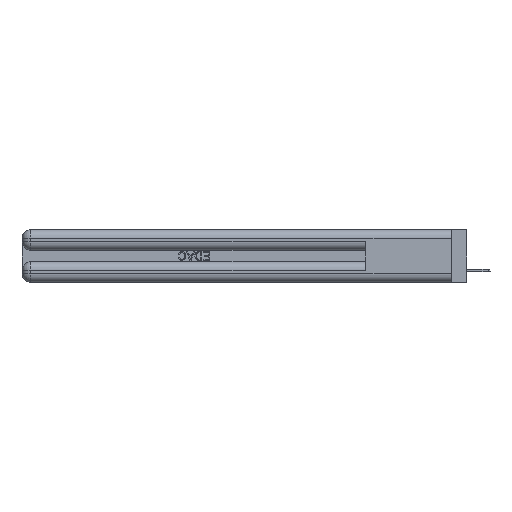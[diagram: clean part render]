
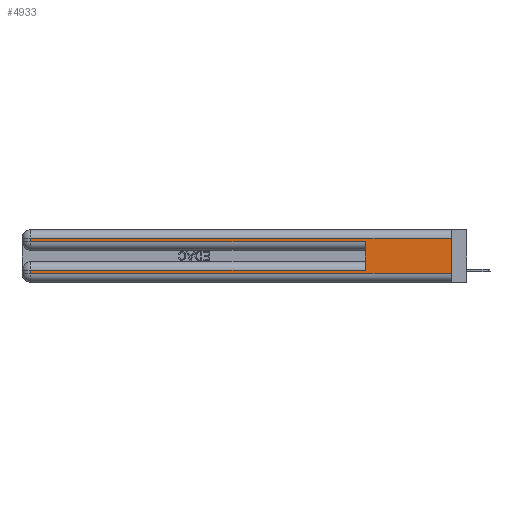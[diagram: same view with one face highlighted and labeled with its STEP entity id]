
A CAD part, left-side view. The second image highlights one B-rep face of the part: STEP entity #4933.
In plain terms, the highlighted planar face has unit normal (-1, 0, 0).
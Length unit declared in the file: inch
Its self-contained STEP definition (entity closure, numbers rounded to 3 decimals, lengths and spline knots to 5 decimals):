
#1 = FACE_OUTER_BOUND ( 'NONE', #5057, .T. ) ;
#409 = VERTEX_POINT ( 'NONE', #12928 ) ;
#585 = VERTEX_POINT ( 'NONE', #13416 ) ;
#693 = EDGE_CURVE ( 'NONE', #15766, #15949, #33570, .T. ) ;
#899 = VECTOR ( 'NONE', #7344, 39.37008 ) ;
#920 = ORIENTED_EDGE ( 'NONE', *, *, #13534, .T. ) ;
#3153 = ORIENTED_EDGE ( 'NONE', *, *, #22702, .F. ) ;
#3956 = DIRECTION ( 'NONE',  ( 0., 0., 1. ) ) ;
#4933 = ADVANCED_FACE ( 'NONE', ( #1 ), #30703, .F. ) ;
#5057 = EDGE_LOOP ( 'NONE', ( #3153, #31452, #42704, #10054, #16889, #920, #41786, #15667 ) ) ;
#5672 = CARTESIAN_POINT ( 'NONE',  ( 0., 0., 0.085 ) ) ;
#6010 = VECTOR ( 'NONE', #7551, 39.37008 ) ;
#7015 = EDGE_CURVE ( 'NONE', #585, #23819, #20651, .T. ) ;
#7344 = DIRECTION ( 'NONE',  ( 0., 1., 0. ) ) ;
#7551 = DIRECTION ( 'NONE',  ( 0., 0., -1. ) ) ;
#9021 = LINE ( 'NONE', #29545, #44874 ) ;
#9796 = LINE ( 'NONE', #39107, #19837 ) ;
#10054 = ORIENTED_EDGE ( 'NONE', *, *, #35506, .T. ) ;
#10888 = EDGE_CURVE ( 'NONE', #15949, #28149, #39753, .T. ) ;
#11546 = CARTESIAN_POINT ( 'NONE',  ( 0., 0., 0.06 ) ) ;
#11965 = DIRECTION ( 'NONE',  ( 0., -1., 0. ) ) ;
#12458 = CARTESIAN_POINT ( 'NONE',  ( 0., 0., 0.31 ) ) ;
#12928 = CARTESIAN_POINT ( 'NONE',  ( 0., 2.94, 0.085 ) ) ;
#13416 = CARTESIAN_POINT ( 'NONE',  ( 0., 0.6, 0.085 ) ) ;
#13534 = EDGE_CURVE ( 'NONE', #585, #409, #28419, .T. ) ;
#14005 = CARTESIAN_POINT ( 'NONE',  ( 0., 0., 0.31 ) ) ;
#14333 = CARTESIAN_POINT ( 'NONE',  ( 0., 0.6, 0.145 ) ) ;
#15351 = AXIS2_PLACEMENT_3D ( 'NONE', #30994, #27719, #19470 ) ;
#15667 = ORIENTED_EDGE ( 'NONE', *, *, #41146, .T. ) ;
#15766 = VERTEX_POINT ( 'NONE', #12458 ) ;
#15949 = VERTEX_POINT ( 'NONE', #16830 ) ;
#16182 = VECTOR ( 'NONE', #16986, 39.37008 ) ;
#16830 = CARTESIAN_POINT ( 'NONE',  ( 0., 2.94, 0.31 ) ) ;
#16889 = ORIENTED_EDGE ( 'NONE', *, *, #7015, .F. ) ;
#16986 = DIRECTION ( 'NONE',  ( 0., -1., 0. ) ) ;
#17973 = VECTOR ( 'NONE', #23342, 39.37008 ) ;
#18191 = LINE ( 'NONE', #39471, #6010 ) ;
#19470 = DIRECTION ( 'NONE',  ( 0., 0., -1. ) ) ;
#19837 = VECTOR ( 'NONE', #31599, 39.37008 ) ;
#20651 = LINE ( 'NONE', #14333, #37131 ) ;
#21470 = VERTEX_POINT ( 'NONE', #31205 ) ;
#21498 = CARTESIAN_POINT ( 'NONE',  ( 0., 2.94, 0.37 ) ) ;
#22702 = EDGE_CURVE ( 'NONE', #15766, #26576, #9796, .T. ) ;
#23342 = DIRECTION ( 'NONE',  ( 0., 1., 0. ) ) ;
#23608 = CARTESIAN_POINT ( 'NONE',  ( 0., 0., 0.06 ) ) ;
#23819 = VERTEX_POINT ( 'NONE', #34543 ) ;
#26576 = VERTEX_POINT ( 'NONE', #11546 ) ;
#27719 = DIRECTION ( 'NONE',  ( 1., 0., 0. ) ) ;
#28149 = VERTEX_POINT ( 'NONE', #31568 ) ;
#28419 = LINE ( 'NONE', #5672, #17973 ) ;
#29545 = CARTESIAN_POINT ( 'NONE',  ( 0., 0., 0.285 ) ) ;
#30703 = PLANE ( 'NONE',  #15351 ) ;
#30994 = CARTESIAN_POINT ( 'NONE',  ( 0., 0., 0.37 ) ) ;
#31205 = CARTESIAN_POINT ( 'NONE',  ( 0., 2.94, 0.06 ) ) ;
#31452 = ORIENTED_EDGE ( 'NONE', *, *, #693, .T. ) ;
#31568 = CARTESIAN_POINT ( 'NONE',  ( 0., 2.94, 0.285 ) ) ;
#31599 = DIRECTION ( 'NONE',  ( 0., 0., -1. ) ) ;
#33570 = LINE ( 'NONE', #14005, #899 ) ;
#34543 = CARTESIAN_POINT ( 'NONE',  ( 0., 0.6, 0.285 ) ) ;
#35356 = VECTOR ( 'NONE', #42397, 39.37008 ) ;
#35506 = EDGE_CURVE ( 'NONE', #28149, #23819, #9021, .T. ) ;
#37131 = VECTOR ( 'NONE', #3956, 39.37008 ) ;
#39107 = CARTESIAN_POINT ( 'NONE',  ( 0., 0., 0.37 ) ) ;
#39471 = CARTESIAN_POINT ( 'NONE',  ( 0., 2.94, 0.37 ) ) ;
#39753 = LINE ( 'NONE', #21498, #35356 ) ;
#41146 = EDGE_CURVE ( 'NONE', #21470, #26576, #41493, .T. ) ;
#41493 = LINE ( 'NONE', #23608, #16182 ) ;
#41786 = ORIENTED_EDGE ( 'NONE', *, *, #44179, .T. ) ;
#42397 = DIRECTION ( 'NONE',  ( 0., 0., -1. ) ) ;
#42704 = ORIENTED_EDGE ( 'NONE', *, *, #10888, .T. ) ;
#44179 = EDGE_CURVE ( 'NONE', #409, #21470, #18191, .T. ) ;
#44874 = VECTOR ( 'NONE', #11965, 39.37008 ) ;
